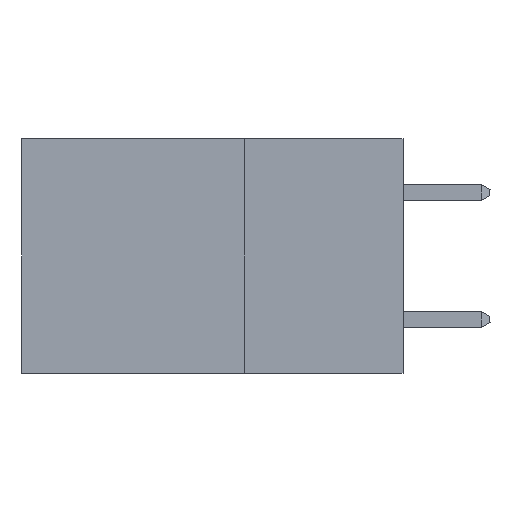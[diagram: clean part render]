
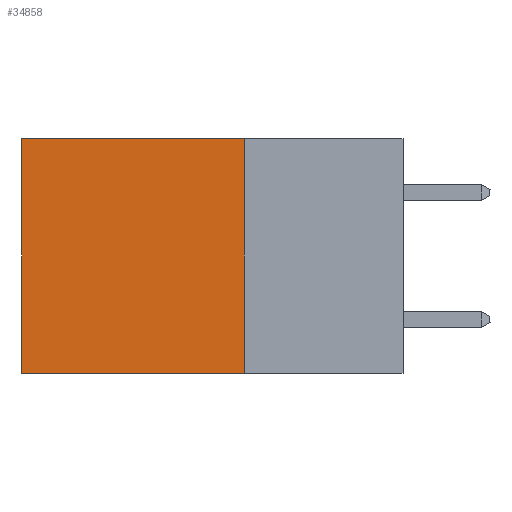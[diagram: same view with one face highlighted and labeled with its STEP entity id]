
A CAD part, left-side view. The second image highlights one B-rep face of the part: STEP entity #34858.
In plain terms, the highlighted planar face has unit normal (-1, 0, 0).
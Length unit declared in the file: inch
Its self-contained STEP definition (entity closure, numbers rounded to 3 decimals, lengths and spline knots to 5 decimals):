
#1726 = ORIENTED_EDGE ( 'NONE', *, *, #43486, .T. ) ;
#2690 = ORIENTED_EDGE ( 'NONE', *, *, #41812, .T. ) ;
#2911 = DIRECTION ( 'NONE',  ( 0., 1., 0. ) ) ;
#3014 = VERTEX_POINT ( 'NONE', #12013 ) ;
#4019 = EDGE_CURVE ( 'NONE', #25446, #27160, #13075, .T. ) ;
#5695 = VECTOR ( 'NONE', #33792, 39.37008 ) ;
#5993 = EDGE_CURVE ( 'NONE', #27160, #15913, #42854, .T. ) ;
#6573 = CARTESIAN_POINT ( 'NONE',  ( 0.2875, 0.25, 0. ) ) ;
#6653 = DIRECTION ( 'NONE',  ( 0., 0., -1. ) ) ;
#12013 = CARTESIAN_POINT ( 'NONE',  ( 0.2875, 0.6, 0. ) ) ;
#13075 = LINE ( 'NONE', #6573, #32441 ) ;
#15001 = ORIENTED_EDGE ( 'NONE', *, *, #5993, .F. ) ;
#15913 = VERTEX_POINT ( 'NONE', #39671 ) ;
#19194 = CARTESIAN_POINT ( 'NONE',  ( 0.2875, 0.25, -0.37 ) ) ;
#21588 = VECTOR ( 'NONE', #2911, 39.37008 ) ;
#25446 = VERTEX_POINT ( 'NONE', #39349 ) ;
#25690 = ORIENTED_EDGE ( 'NONE', *, *, #4019, .F. ) ;
#25776 = CARTESIAN_POINT ( 'NONE',  ( 0.2875, 0.25, 0. ) ) ;
#27160 = VERTEX_POINT ( 'NONE', #42300 ) ;
#30619 = PLANE ( 'NONE',  #49853 ) ;
#32441 = VECTOR ( 'NONE', #34538, 39.37008 ) ;
#33792 = DIRECTION ( 'NONE',  ( 0., 1., 0. ) ) ;
#34538 = DIRECTION ( 'NONE',  ( 0., 0., -1. ) ) ;
#34803 = CARTESIAN_POINT ( 'NONE',  ( 0.2875, 0.25, 0. ) ) ;
#34858 = ADVANCED_FACE ( 'NONE', ( #51738 ), #30619, .F. ) ;
#34913 = VECTOR ( 'NONE', #48224, 39.37008 ) ;
#35113 = LINE ( 'NONE', #25776, #5695 ) ;
#35633 = EDGE_LOOP ( 'NONE', ( #1726, #15001, #25690, #2690 ) ) ;
#38463 = DIRECTION ( 'NONE',  ( 1., 0., 0. ) ) ;
#39349 = CARTESIAN_POINT ( 'NONE',  ( 0.2875, 0.25, 0. ) ) ;
#39671 = CARTESIAN_POINT ( 'NONE',  ( 0.2875, 0.6, -0.37 ) ) ;
#41812 = EDGE_CURVE ( 'NONE', #25446, #3014, #35113, .T. ) ;
#42300 = CARTESIAN_POINT ( 'NONE',  ( 0.2875, 0.25, -0.37 ) ) ;
#42854 = LINE ( 'NONE', #19194, #21588 ) ;
#43486 = EDGE_CURVE ( 'NONE', #3014, #15913, #46851, .T. ) ;
#46851 = LINE ( 'NONE', #51719, #34913 ) ;
#48224 = DIRECTION ( 'NONE',  ( 0., 0., -1. ) ) ;
#49853 = AXIS2_PLACEMENT_3D ( 'NONE', #34803, #38463, #6653 ) ;
#51719 = CARTESIAN_POINT ( 'NONE',  ( 0.2875, 0.6, 0. ) ) ;
#51738 = FACE_OUTER_BOUND ( 'NONE', #35633, .T. ) ;
